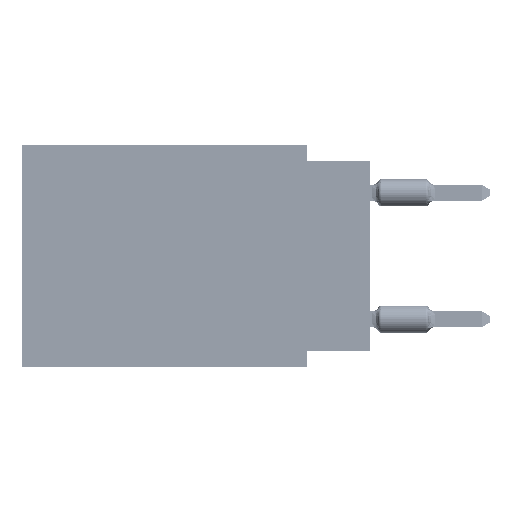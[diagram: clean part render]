
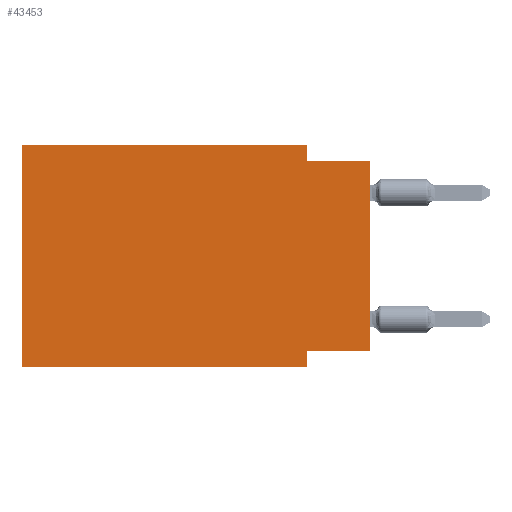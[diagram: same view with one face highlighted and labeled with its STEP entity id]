
A CAD part, left-side view. The second image highlights one B-rep face of the part: STEP entity #43453.
In plain terms, the highlighted planar face has unit normal (-1, 0, 0).
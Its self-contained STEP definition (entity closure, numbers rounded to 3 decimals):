
#1937 = VERTEX_POINT ( 'NONE', #81893 ) ;
#2550 = AXIS2_PLACEMENT_3D ( 'NONE', #21057, #12894, #37942 ) ;
#4694 = PLANE ( 'NONE',  #2550 ) ;
#5912 = DIRECTION ( 'NONE',  ( 0., 0., 1. ) ) ;
#6444 = LINE ( 'NONE', #95366, #86136 ) ;
#7922 = CARTESIAN_POINT ( 'NONE',  ( 0., 0., 0. ) ) ;
#11305 = DIRECTION ( 'NONE',  ( 0., -1., 0. ) ) ;
#11708 = VECTOR ( 'NONE', #79297, 1000. ) ;
#11729 = ORIENTED_EDGE ( 'NONE', *, *, #44811, .F. ) ;
#12874 = CARTESIAN_POINT ( 'NONE',  ( 0., 2.54, -8.255 ) ) ;
#12894 = DIRECTION ( 'NONE',  ( 1., 0., 0. ) ) ;
#14009 = EDGE_CURVE ( 'NONE', #55081, #27151, #103844, .T. ) ;
#15503 = EDGE_CURVE ( 'NONE', #82562, #1937, #102874, .T. ) ;
#15963 = EDGE_CURVE ( 'NONE', #21868, #99402, #96199, .T. ) ;
#16424 = ORIENTED_EDGE ( 'NONE', *, *, #60287, .F. ) ;
#16837 = CARTESIAN_POINT ( 'NONE',  ( 0., 13.97, -8.89 ) ) ;
#18196 = ORIENTED_EDGE ( 'NONE', *, *, #102938, .F. ) ;
#19172 = EDGE_LOOP ( 'NONE', ( #51444, #39408, #18196, #22869, #11729, #55507, #103180, #16424 ) ) ;
#20963 = CARTESIAN_POINT ( 'NONE',  ( 0., 13.97, 0. ) ) ;
#21057 = CARTESIAN_POINT ( 'NONE',  ( 0., 13.97, 0. ) ) ;
#21868 = VERTEX_POINT ( 'NONE', #16837 ) ;
#21870 = CARTESIAN_POINT ( 'NONE',  ( 0., 0., -8.255 ) ) ;
#22720 = VECTOR ( 'NONE', #80633, 1000. ) ;
#22869 = ORIENTED_EDGE ( 'NONE', *, *, #14009, .F. ) ;
#24430 = EDGE_CURVE ( 'NONE', #61781, #1937, #41692, .T. ) ;
#25378 = CARTESIAN_POINT ( 'NONE',  ( 0., 13.97, 0. ) ) ;
#26715 = VECTOR ( 'NONE', #104911, 1000. ) ;
#27151 = VERTEX_POINT ( 'NONE', #84446 ) ;
#27663 = CARTESIAN_POINT ( 'NONE',  ( 0., 2.54, -0.635 ) ) ;
#29255 = FACE_OUTER_BOUND ( 'NONE', #19172, .T. ) ;
#32835 = CARTESIAN_POINT ( 'NONE',  ( 0., 2.54, -8.89 ) ) ;
#37942 = DIRECTION ( 'NONE',  ( 0., 0., -1. ) ) ;
#39408 = ORIENTED_EDGE ( 'NONE', *, *, #15503, .F. ) ;
#40430 = LINE ( 'NONE', #90588, #64791 ) ;
#40989 = LINE ( 'NONE', #74252, #49964 ) ;
#41692 = LINE ( 'NONE', #7922, #94258 ) ;
#43453 = ADVANCED_FACE ( 'NONE', ( #29255 ), #4694, .F. ) ;
#44811 = EDGE_CURVE ( 'NONE', #21868, #55081, #6444, .T. ) ;
#48221 = VECTOR ( 'NONE', #11305, 1000. ) ;
#49964 = VECTOR ( 'NONE', #107507, 1000. ) ;
#51444 = ORIENTED_EDGE ( 'NONE', *, *, #24430, .T. ) ;
#52097 = EDGE_CURVE ( 'NONE', #86430, #99402, #63220, .T. ) ;
#52727 = CARTESIAN_POINT ( 'NONE',  ( 0., 0., -0.635 ) ) ;
#55081 = VERTEX_POINT ( 'NONE', #25378 ) ;
#55507 = ORIENTED_EDGE ( 'NONE', *, *, #15963, .T. ) ;
#60287 = EDGE_CURVE ( 'NONE', #61781, #86430, #40989, .T. ) ;
#61781 = VERTEX_POINT ( 'NONE', #21870 ) ;
#63220 = LINE ( 'NONE', #90949, #22720 ) ;
#64791 = VECTOR ( 'NONE', #65529, 1000. ) ;
#65529 = DIRECTION ( 'NONE',  ( 0., 0., -1. ) ) ;
#74252 = CARTESIAN_POINT ( 'NONE',  ( 0., 0., -8.255 ) ) ;
#79297 = DIRECTION ( 'NONE',  ( 0., -1., 0. ) ) ;
#79811 = CARTESIAN_POINT ( 'NONE',  ( 0., 13.97, -8.89 ) ) ;
#80633 = DIRECTION ( 'NONE',  ( 0., 0., -1. ) ) ;
#81893 = CARTESIAN_POINT ( 'NONE',  ( 0., 0., -0.635 ) ) ;
#82562 = VERTEX_POINT ( 'NONE', #27663 ) ;
#84446 = CARTESIAN_POINT ( 'NONE',  ( 0., 2.54, 0. ) ) ;
#86136 = VECTOR ( 'NONE', #5912, 1000. ) ;
#86430 = VERTEX_POINT ( 'NONE', #12874 ) ;
#90588 = CARTESIAN_POINT ( 'NONE',  ( 0., 2.54, 0. ) ) ;
#90949 = CARTESIAN_POINT ( 'NONE',  ( 0., 2.54, -8.89 ) ) ;
#91332 = DIRECTION ( 'NONE',  ( 0., 0., 1. ) ) ;
#94258 = VECTOR ( 'NONE', #91332, 1000. ) ;
#95366 = CARTESIAN_POINT ( 'NONE',  ( 0., 13.97, 0. ) ) ;
#96199 = LINE ( 'NONE', #79811, #11708 ) ;
#99402 = VERTEX_POINT ( 'NONE', #32835 ) ;
#102874 = LINE ( 'NONE', #52727, #48221 ) ;
#102938 = EDGE_CURVE ( 'NONE', #27151, #82562, #40430, .T. ) ;
#103180 = ORIENTED_EDGE ( 'NONE', *, *, #52097, .F. ) ;
#103844 = LINE ( 'NONE', #20963, #26715 ) ;
#104911 = DIRECTION ( 'NONE',  ( 0., -1., 0. ) ) ;
#107507 = DIRECTION ( 'NONE',  ( 0., 1., 0. ) ) ;
